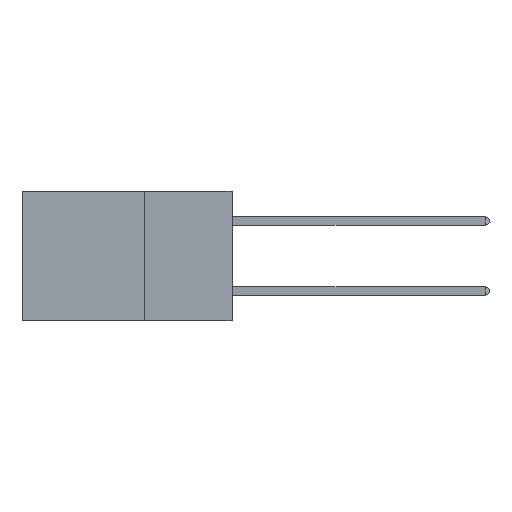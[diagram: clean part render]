
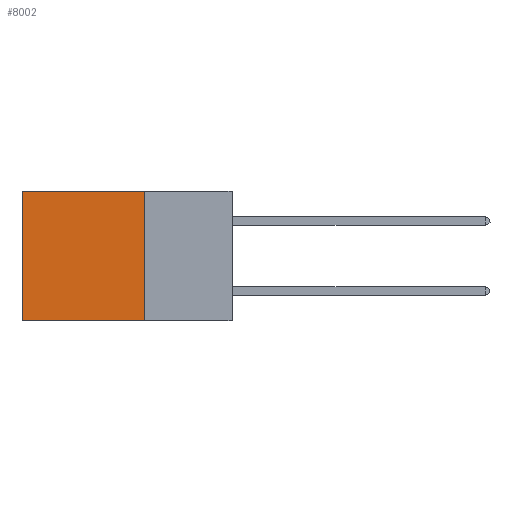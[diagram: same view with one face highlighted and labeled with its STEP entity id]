
A CAD part, left-side view. The second image highlights one B-rep face of the part: STEP entity #8002.
In plain terms, the highlighted planar face has unit normal (-1, 0, 0).
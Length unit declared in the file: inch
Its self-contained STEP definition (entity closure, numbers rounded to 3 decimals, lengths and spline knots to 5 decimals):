
#1572 = CARTESIAN_POINT ( 'NONE',  ( 0.2875, 0.25, -0.37 ) ) ;
#1644 = CARTESIAN_POINT ( 'NONE',  ( 0.2875, 0.6, 0. ) ) ;
#1699 = AXIS2_PLACEMENT_3D ( 'NONE', #6181, #17642, #12974 ) ;
#2183 = VECTOR ( 'NONE', #12337, 39.37008 ) ;
#4710 = VERTEX_POINT ( 'NONE', #1572 ) ;
#4914 = LINE ( 'NONE', #11071, #16578 ) ;
#5366 = VECTOR ( 'NONE', #13501, 39.37008 ) ;
#5415 = EDGE_CURVE ( 'NONE', #12809, #4710, #4914, .T. ) ;
#6181 = CARTESIAN_POINT ( 'NONE',  ( 0.2875, 0.25, 0. ) ) ;
#6185 = DIRECTION ( 'NONE',  ( 0., 0., -1. ) ) ;
#7383 = EDGE_LOOP ( 'NONE', ( #11227, #9503, #21157, #14538 ) ) ;
#7840 = CARTESIAN_POINT ( 'NONE',  ( 0.2875, 0.25, 0. ) ) ;
#7856 = EDGE_CURVE ( 'NONE', #12395, #15764, #9988, .T. ) ;
#7889 = LINE ( 'NONE', #17002, #20089 ) ;
#8002 = ADVANCED_FACE ( 'NONE', ( #14185 ), #15224, .F. ) ;
#8117 = EDGE_CURVE ( 'NONE', #12809, #12395, #16266, .T. ) ;
#9503 = ORIENTED_EDGE ( 'NONE', *, *, #11190, .F. ) ;
#9988 = LINE ( 'NONE', #14088, #2183 ) ;
#10375 = DIRECTION ( 'NONE',  ( 0., 1., 0. ) ) ;
#11071 = CARTESIAN_POINT ( 'NONE',  ( 0.2875, 0.25, 0. ) ) ;
#11190 = EDGE_CURVE ( 'NONE', #4710, #15764, #7889, .T. ) ;
#11227 = ORIENTED_EDGE ( 'NONE', *, *, #7856, .T. ) ;
#12337 = DIRECTION ( 'NONE',  ( 0., 0., -1. ) ) ;
#12395 = VERTEX_POINT ( 'NONE', #1644 ) ;
#12809 = VERTEX_POINT ( 'NONE', #7840 ) ;
#12974 = DIRECTION ( 'NONE',  ( 0., 0., -1. ) ) ;
#13501 = DIRECTION ( 'NONE',  ( 0., 1., 0. ) ) ;
#14088 = CARTESIAN_POINT ( 'NONE',  ( 0.2875, 0.6, 0. ) ) ;
#14185 = FACE_OUTER_BOUND ( 'NONE', #7383, .T. ) ;
#14538 = ORIENTED_EDGE ( 'NONE', *, *, #8117, .T. ) ;
#15224 = PLANE ( 'NONE',  #1699 ) ;
#15764 = VERTEX_POINT ( 'NONE', #18606 ) ;
#16266 = LINE ( 'NONE', #20302, #5366 ) ;
#16578 = VECTOR ( 'NONE', #6185, 39.37008 ) ;
#17002 = CARTESIAN_POINT ( 'NONE',  ( 0.2875, 0.25, -0.37 ) ) ;
#17642 = DIRECTION ( 'NONE',  ( 1., 0., 0. ) ) ;
#18606 = CARTESIAN_POINT ( 'NONE',  ( 0.2875, 0.6, -0.37 ) ) ;
#20089 = VECTOR ( 'NONE', #10375, 39.37008 ) ;
#20302 = CARTESIAN_POINT ( 'NONE',  ( 0.2875, 0.25, 0. ) ) ;
#21157 = ORIENTED_EDGE ( 'NONE', *, *, #5415, .F. ) ;
